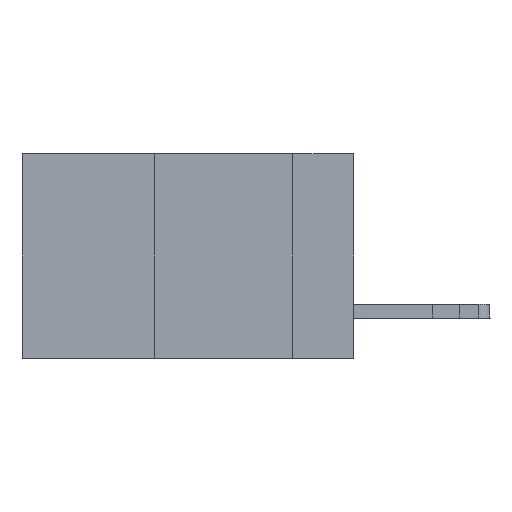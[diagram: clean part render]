
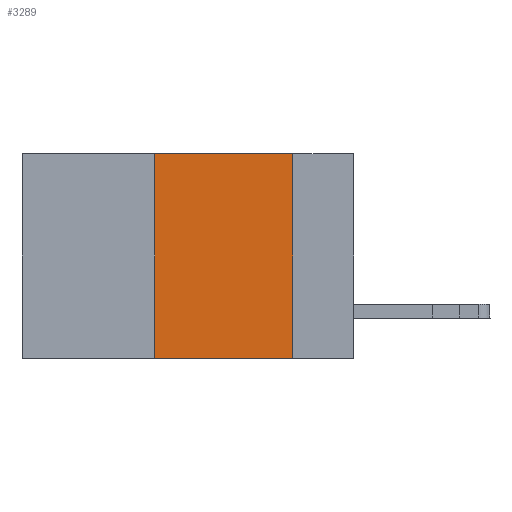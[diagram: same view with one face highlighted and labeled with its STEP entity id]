
A CAD part, left-side view. The second image highlights one B-rep face of the part: STEP entity #3289.
In plain terms, the highlighted planar face has unit normal (-1, 0, 0).
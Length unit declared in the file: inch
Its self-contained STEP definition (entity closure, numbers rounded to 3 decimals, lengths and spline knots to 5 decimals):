
#149 = DIRECTION ( 'NONE',  ( 0., -1., 0. ) ) ;
#555 = VECTOR ( 'NONE', #11492, 39.37008 ) ;
#1318 = CARTESIAN_POINT ( 'NONE',  ( 0., 0.6, -0.37 ) ) ;
#1768 = EDGE_CURVE ( 'NONE', #17944, #17753, #5622, .T. ) ;
#1867 = PLANE ( 'NONE',  #3294 ) ;
#2127 = VECTOR ( 'NONE', #149, 39.37008 ) ;
#2135 = VERTEX_POINT ( 'NONE', #12210 ) ;
#2836 = LINE ( 'NONE', #15487, #13404 ) ;
#3037 = CARTESIAN_POINT ( 'NONE',  ( 0., 0.36, -0.37 ) ) ;
#3289 = ADVANCED_FACE ( 'NONE', ( #11595 ), #1867, .F. ) ;
#3294 = AXIS2_PLACEMENT_3D ( 'NONE', #4904, #9115, #7572 ) ;
#4904 = CARTESIAN_POINT ( 'NONE',  ( 0., 0.6, 0. ) ) ;
#5622 = LINE ( 'NONE', #1318, #555 ) ;
#6173 = ORIENTED_EDGE ( 'NONE', *, *, #6255, .F. ) ;
#6255 = EDGE_CURVE ( 'NONE', #9333, #17753, #2836, .T. ) ;
#6898 = CARTESIAN_POINT ( 'NONE',  ( 0., 0.36, 0. ) ) ;
#7572 = DIRECTION ( 'NONE',  ( 0., 0., -1. ) ) ;
#8551 = EDGE_CURVE ( 'NONE', #17944, #2135, #13845, .T. ) ;
#8712 = DIRECTION ( 'NONE',  ( 0., 0., -1. ) ) ;
#9115 = DIRECTION ( 'NONE',  ( 1., 0., 0. ) ) ;
#9333 = VERTEX_POINT ( 'NONE', #15898 ) ;
#9872 = ORIENTED_EDGE ( 'NONE', *, *, #15224, .F. ) ;
#11425 = LINE ( 'NONE', #15454, #2127 ) ;
#11492 = DIRECTION ( 'NONE',  ( 0., -1., 0. ) ) ;
#11595 = FACE_OUTER_BOUND ( 'NONE', #17288, .T. ) ;
#12210 = CARTESIAN_POINT ( 'NONE',  ( 0., 0.36, 0. ) ) ;
#12813 = VECTOR ( 'NONE', #15129, 39.37008 ) ;
#13404 = VECTOR ( 'NONE', #8712, 39.37008 ) ;
#13845 = LINE ( 'NONE', #6898, #12813 ) ;
#15129 = DIRECTION ( 'NONE',  ( 0., 0., 1. ) ) ;
#15224 = EDGE_CURVE ( 'NONE', #2135, #9333, #11425, .T. ) ;
#15454 = CARTESIAN_POINT ( 'NONE',  ( 0., 0.6, 0. ) ) ;
#15487 = CARTESIAN_POINT ( 'NONE',  ( 0., 0.11, 0. ) ) ;
#15898 = CARTESIAN_POINT ( 'NONE',  ( 0., 0.11, 0. ) ) ;
#16565 = ORIENTED_EDGE ( 'NONE', *, *, #1768, .T. ) ;
#17130 = ORIENTED_EDGE ( 'NONE', *, *, #8551, .F. ) ;
#17288 = EDGE_LOOP ( 'NONE', ( #6173, #9872, #17130, #16565 ) ) ;
#17753 = VERTEX_POINT ( 'NONE', #18050 ) ;
#17944 = VERTEX_POINT ( 'NONE', #3037 ) ;
#18050 = CARTESIAN_POINT ( 'NONE',  ( 0., 0.11, -0.37 ) ) ;
